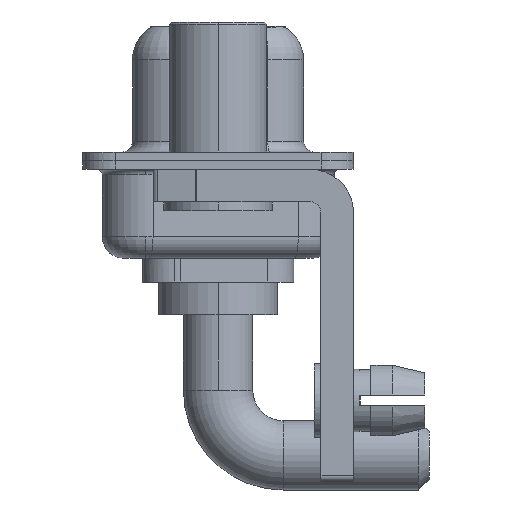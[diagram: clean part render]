
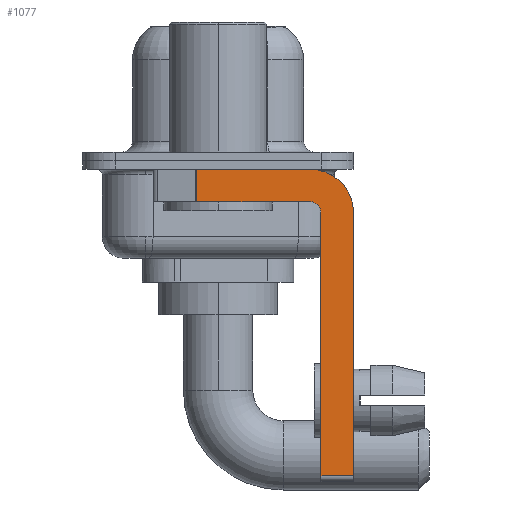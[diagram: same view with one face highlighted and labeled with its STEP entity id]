
A CAD part, left-side view. The second image highlights one B-rep face of the part: STEP entity #1077.
In plain terms, the highlighted planar face has unit normal (-1, 0, 0).
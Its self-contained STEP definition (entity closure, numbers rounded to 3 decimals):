
#303 = CARTESIAN_POINT ( 'NONE',  ( -2.9, -4.25, -0.4 ) ) ;
#338 = VERTEX_POINT ( 'NONE', #303 ) ;
#549 = CARTESIAN_POINT ( 'NONE',  ( -2.9, -6.25, -14.55 ) ) ;
#597 = AXIS2_PLACEMENT_3D ( 'NONE', #3964, #14433, #10775 ) ;
#974 = CARTESIAN_POINT ( 'NONE',  ( -2.9, 3., -0.4 ) ) ;
#1044 = CARTESIAN_POINT ( 'NONE',  ( -2.9, -4.25, -2.4 ) ) ;
#1077 = ADVANCED_FACE ( 'NONE', ( #12986 ), #2669, .F. ) ;
#1129 = EDGE_CURVE ( 'NONE', #7422, #4066, #1305, .T. ) ;
#1305 = LINE ( 'NONE', #6524, #1356 ) ;
#1356 = VECTOR ( 'NONE', #6261, 1000. ) ;
#1568 = LINE ( 'NONE', #6786, #10122 ) ;
#1862 = CARTESIAN_POINT ( 'NONE',  ( -2.9, 0.978, -1.9 ) ) ;
#2053 = CARTESIAN_POINT ( 'NONE',  ( -2.9, -6.25, -2.4 ) ) ;
#2209 = ORIENTED_EDGE ( 'NONE', *, *, #1129, .F. ) ;
#2669 = PLANE ( 'NONE',  #6541 ) ;
#3130 = EDGE_CURVE ( 'NONE', #15700, #12179, #8062, .T. ) ;
#3159 = DIRECTION ( 'NONE',  ( -1., 0., 0. ) ) ;
#3184 = ORIENTED_EDGE ( 'NONE', *, *, #14833, .T. ) ;
#3321 = CARTESIAN_POINT ( 'NONE',  ( -2.9, -4.25, -2.4 ) ) ;
#3964 = CARTESIAN_POINT ( 'NONE',  ( -2.9, -4.25, -2.4 ) ) ;
#4059 = CARTESIAN_POINT ( 'NONE',  ( -2.9, -4.25, -1.9 ) ) ;
#4066 = VERTEX_POINT ( 'NONE', #549 ) ;
#4718 = DIRECTION ( 'NONE',  ( 0., 1., 0. ) ) ;
#4902 = LINE ( 'NONE', #974, #12060 ) ;
#4928 = EDGE_CURVE ( 'NONE', #338, #7422, #9855, .T. ) ;
#5643 = CARTESIAN_POINT ( 'NONE',  ( -2.9, -4.75, -14.8 ) ) ;
#5969 = ORIENTED_EDGE ( 'NONE', *, *, #6280, .F. ) ;
#6261 = DIRECTION ( 'NONE',  ( 0., 0., -1. ) ) ;
#6280 = EDGE_CURVE ( 'NONE', #15480, #338, #4902, .T. ) ;
#6524 = CARTESIAN_POINT ( 'NONE',  ( -2.9, -6.25, -2.4 ) ) ;
#6541 = AXIS2_PLACEMENT_3D ( 'NONE', #1044, #11789, #7887 ) ;
#6598 = EDGE_CURVE ( 'NONE', #12179, #12105, #11195, .T. ) ;
#6699 = DIRECTION ( 'NONE',  ( 0., -1., 0. ) ) ;
#6786 = CARTESIAN_POINT ( 'NONE',  ( -2.9, -4.25, -14.55 ) ) ;
#7422 = VERTEX_POINT ( 'NONE', #2053 ) ;
#7887 = DIRECTION ( 'NONE',  ( 0., 0., -1. ) ) ;
#7924 = VECTOR ( 'NONE', #4718, 1000. ) ;
#8062 = CIRCLE ( 'NONE', #12681, 0.5 ) ;
#8131 = EDGE_CURVE ( 'NONE', #13338, #4066, #1568, .T. ) ;
#8269 = VECTOR ( 'NONE', #13227, 1000. ) ;
#9855 = CIRCLE ( 'NONE', #597, 2. ) ;
#9971 = DIRECTION ( 'NONE',  ( 0., 0., 1. ) ) ;
#10122 = VECTOR ( 'NONE', #6699, 1000. ) ;
#10306 = ORIENTED_EDGE ( 'NONE', *, *, #3130, .F. ) ;
#10775 = DIRECTION ( 'NONE',  ( 0., 0., -1. ) ) ;
#10843 = CARTESIAN_POINT ( 'NONE',  ( -2.9, -4.75, -2.4 ) ) ;
#10962 = CARTESIAN_POINT ( 'NONE',  ( -2.9, -4.75, -14.55 ) ) ;
#11066 = ORIENTED_EDGE ( 'NONE', *, *, #4928, .F. ) ;
#11195 = LINE ( 'NONE', #16400, #7924 ) ;
#11789 = DIRECTION ( 'NONE',  ( 1., 0., 0. ) ) ;
#12060 = VECTOR ( 'NONE', #12910, 1000. ) ;
#12097 = LINE ( 'NONE', #1862, #15516 ) ;
#12105 = VERTEX_POINT ( 'NONE', #14366 ) ;
#12179 = VERTEX_POINT ( 'NONE', #4059 ) ;
#12681 = AXIS2_PLACEMENT_3D ( 'NONE', #3321, #3159, #9971 ) ;
#12910 = DIRECTION ( 'NONE',  ( 0., -1., 0. ) ) ;
#12986 = FACE_OUTER_BOUND ( 'NONE', #16228, .T. ) ;
#13227 = DIRECTION ( 'NONE',  ( 0., 0., 1. ) ) ;
#13338 = VERTEX_POINT ( 'NONE', #10962 ) ;
#14277 = EDGE_CURVE ( 'NONE', #13338, #15700, #15964, .T. ) ;
#14286 = ORIENTED_EDGE ( 'NONE', *, *, #14277, .F. ) ;
#14366 = CARTESIAN_POINT ( 'NONE',  ( -2.9, 0.978, -1.9 ) ) ;
#14433 = DIRECTION ( 'NONE',  ( 1., 0., 0. ) ) ;
#14823 = DIRECTION ( 'NONE',  ( 0., 0., -1. ) ) ;
#14833 = EDGE_CURVE ( 'NONE', #15480, #12105, #12097, .T. ) ;
#15377 = CARTESIAN_POINT ( 'NONE',  ( -2.9, 0.978, -0.4 ) ) ;
#15480 = VERTEX_POINT ( 'NONE', #15377 ) ;
#15516 = VECTOR ( 'NONE', #14823, 1000. ) ;
#15700 = VERTEX_POINT ( 'NONE', #10843 ) ;
#15964 = LINE ( 'NONE', #5643, #8269 ) ;
#15977 = ORIENTED_EDGE ( 'NONE', *, *, #8131, .T. ) ;
#16228 = EDGE_LOOP ( 'NONE', ( #5969, #3184, #16609, #10306, #14286, #15977, #2209, #11066 ) ) ;
#16400 = CARTESIAN_POINT ( 'NONE',  ( -2.9, -4.25, -1.9 ) ) ;
#16609 = ORIENTED_EDGE ( 'NONE', *, *, #6598, .F. ) ;
